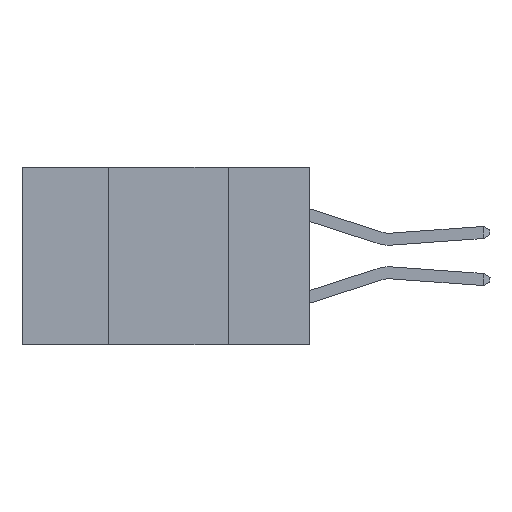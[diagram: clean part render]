
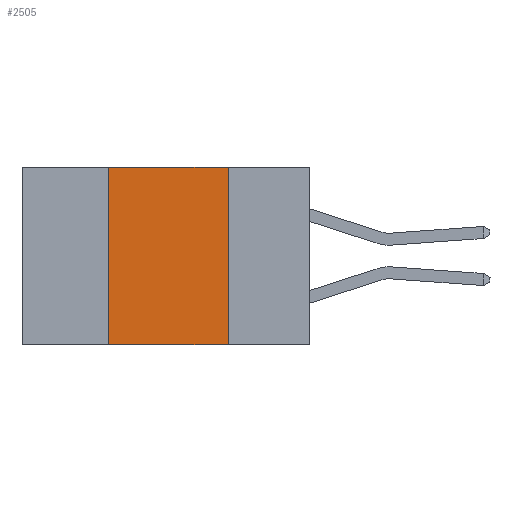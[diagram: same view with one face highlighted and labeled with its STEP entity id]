
A CAD part, left-side view. The second image highlights one B-rep face of the part: STEP entity #2505.
In plain terms, the highlighted planar face has unit normal (-1, 0, 0).
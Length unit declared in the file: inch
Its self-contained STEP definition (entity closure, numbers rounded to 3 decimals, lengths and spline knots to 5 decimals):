
#502 = ORIENTED_EDGE ( 'NONE', *, *, #20515, .T. ) ;
#1116 = LINE ( 'NONE', #8945, #33975 ) ;
#1494 = VERTEX_POINT ( 'NONE', #29123 ) ;
#2370 = CARTESIAN_POINT ( 'NONE',  ( 0., 0.17, 0. ) ) ;
#2505 = ADVANCED_FACE ( 'NONE', ( #2707 ), #2998, .F. ) ;
#2707 = FACE_OUTER_BOUND ( 'NONE', #19378, .T. ) ;
#2998 = PLANE ( 'NONE',  #28175 ) ;
#4862 = VERTEX_POINT ( 'NONE', #8106 ) ;
#5089 = LINE ( 'NONE', #25938, #28097 ) ;
#5859 = ORIENTED_EDGE ( 'NONE', *, *, #9581, .F. ) ;
#6182 = DIRECTION ( 'NONE',  ( 0., 0., -1. ) ) ;
#6248 = ORIENTED_EDGE ( 'NONE', *, *, #18681, .F. ) ;
#8106 = CARTESIAN_POINT ( 'NONE',  ( 0., 0.42, -0.37 ) ) ;
#8945 = CARTESIAN_POINT ( 'NONE',  ( 0., 0.17, 0. ) ) ;
#9581 = EDGE_CURVE ( 'NONE', #4862, #1494, #30986, .T. ) ;
#10187 = VERTEX_POINT ( 'NONE', #2370 ) ;
#10502 = VERTEX_POINT ( 'NONE', #16036 ) ;
#13106 = ORIENTED_EDGE ( 'NONE', *, *, #24978, .F. ) ;
#13215 = CARTESIAN_POINT ( 'NONE',  ( 0., 0.6, -0.37 ) ) ;
#13719 = DIRECTION ( 'NONE',  ( 0., 0., 1. ) ) ;
#13896 = DIRECTION ( 'NONE',  ( 1., 0., 0. ) ) ;
#16036 = CARTESIAN_POINT ( 'NONE',  ( 0., 0.17, -0.37 ) ) ;
#18681 = EDGE_CURVE ( 'NONE', #10187, #10502, #1116, .T. ) ;
#19378 = EDGE_LOOP ( 'NONE', ( #6248, #13106, #5859, #502 ) ) ;
#20515 = EDGE_CURVE ( 'NONE', #4862, #10502, #26892, .T. ) ;
#21637 = DIRECTION ( 'NONE',  ( 0., 0., -1. ) ) ;
#21874 = CARTESIAN_POINT ( 'NONE',  ( 0., 0.42, 0. ) ) ;
#24978 = EDGE_CURVE ( 'NONE', #1494, #10187, #5089, .T. ) ;
#25648 = VECTOR ( 'NONE', #29058, 39.37008 ) ;
#25938 = CARTESIAN_POINT ( 'NONE',  ( 0., 0.6, 0. ) ) ;
#26892 = LINE ( 'NONE', #13215, #25648 ) ;
#27710 = VECTOR ( 'NONE', #13719, 39.37008 ) ;
#28097 = VECTOR ( 'NONE', #31312, 39.37008 ) ;
#28175 = AXIS2_PLACEMENT_3D ( 'NONE', #29622, #13896, #21637 ) ;
#29058 = DIRECTION ( 'NONE',  ( 0., -1., 0. ) ) ;
#29123 = CARTESIAN_POINT ( 'NONE',  ( 0., 0.42, 0. ) ) ;
#29622 = CARTESIAN_POINT ( 'NONE',  ( 0., 0.6, 0. ) ) ;
#30986 = LINE ( 'NONE', #21874, #27710 ) ;
#31312 = DIRECTION ( 'NONE',  ( 0., -1., 0. ) ) ;
#33975 = VECTOR ( 'NONE', #6182, 39.37008 ) ;
